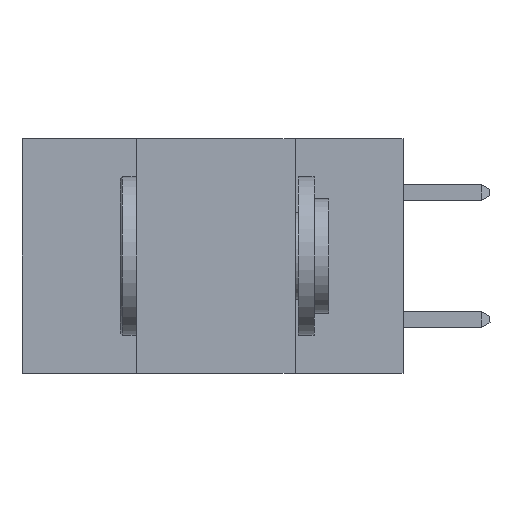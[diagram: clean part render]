
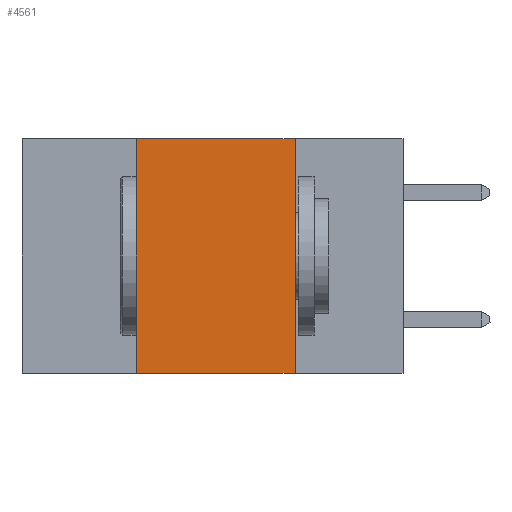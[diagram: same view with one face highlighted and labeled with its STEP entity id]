
A CAD part, left-side view. The second image highlights one B-rep face of the part: STEP entity #4561.
In plain terms, the highlighted planar face has unit normal (-1, 0, 0).
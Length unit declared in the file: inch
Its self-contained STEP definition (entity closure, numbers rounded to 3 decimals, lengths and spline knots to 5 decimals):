
#282 = CARTESIAN_POINT ( 'NONE',  ( 0., 0.6, -0.37 ) ) ;
#1349 = ORIENTED_EDGE ( 'NONE', *, *, #15470, .F. ) ;
#1465 = EDGE_CURVE ( 'NONE', #3434, #4139, #14599, .T. ) ;
#1750 = CARTESIAN_POINT ( 'NONE',  ( 0., 0.42, -0.37 ) ) ;
#2523 = ORIENTED_EDGE ( 'NONE', *, *, #14171, .F. ) ;
#3114 = CARTESIAN_POINT ( 'NONE',  ( 0., 0.17, 0. ) ) ;
#3399 = DIRECTION ( 'NONE',  ( 0., 0., -1. ) ) ;
#3434 = VERTEX_POINT ( 'NONE', #1750 ) ;
#3490 = DIRECTION ( 'NONE',  ( 1., 0., 0. ) ) ;
#3742 = VECTOR ( 'NONE', #6743, 39.37008 ) ;
#3909 = CARTESIAN_POINT ( 'NONE',  ( 0., 0.42, 0. ) ) ;
#4095 = FACE_OUTER_BOUND ( 'NONE', #9824, .T. ) ;
#4135 = LINE ( 'NONE', #282, #3742 ) ;
#4139 = VERTEX_POINT ( 'NONE', #3909 ) ;
#4189 = VECTOR ( 'NONE', #14363, 39.37008 ) ;
#4527 = CARTESIAN_POINT ( 'NONE',  ( 0., 0.17, -0.37 ) ) ;
#4561 = ADVANCED_FACE ( 'NONE', ( #4095 ), #4696, .F. ) ;
#4696 = PLANE ( 'NONE',  #8730 ) ;
#4838 = VERTEX_POINT ( 'NONE', #4527 ) ;
#5543 = VERTEX_POINT ( 'NONE', #3114 ) ;
#5578 = CARTESIAN_POINT ( 'NONE',  ( 0., 0.17, 0. ) ) ;
#6743 = DIRECTION ( 'NONE',  ( 0., -1., 0. ) ) ;
#8730 = AXIS2_PLACEMENT_3D ( 'NONE', #8797, #3490, #3399 ) ;
#8797 = CARTESIAN_POINT ( 'NONE',  ( 0., 0.6, 0. ) ) ;
#9647 = DIRECTION ( 'NONE',  ( 0., -1., 0. ) ) ;
#9824 = EDGE_LOOP ( 'NONE', ( #2523, #1349, #11577, #10497 ) ) ;
#10497 = ORIENTED_EDGE ( 'NONE', *, *, #15224, .T. ) ;
#10675 = LINE ( 'NONE', #14578, #13633 ) ;
#11577 = ORIENTED_EDGE ( 'NONE', *, *, #1465, .F. ) ;
#13108 = VECTOR ( 'NONE', #15478, 39.37008 ) ;
#13633 = VECTOR ( 'NONE', #9647, 39.37008 ) ;
#13971 = CARTESIAN_POINT ( 'NONE',  ( 0., 0.42, 0. ) ) ;
#14171 = EDGE_CURVE ( 'NONE', #5543, #4838, #16225, .T. ) ;
#14363 = DIRECTION ( 'NONE',  ( 0., 0., 1. ) ) ;
#14578 = CARTESIAN_POINT ( 'NONE',  ( 0., 0.6, 0. ) ) ;
#14599 = LINE ( 'NONE', #13971, #4189 ) ;
#15224 = EDGE_CURVE ( 'NONE', #3434, #4838, #4135, .T. ) ;
#15470 = EDGE_CURVE ( 'NONE', #4139, #5543, #10675, .T. ) ;
#15478 = DIRECTION ( 'NONE',  ( 0., 0., -1. ) ) ;
#16225 = LINE ( 'NONE', #5578, #13108 ) ;
